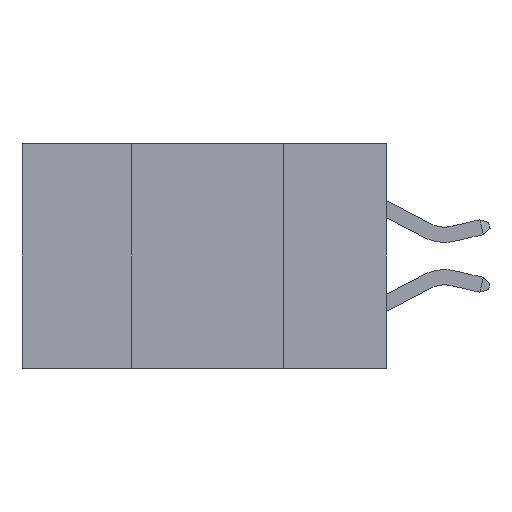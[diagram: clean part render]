
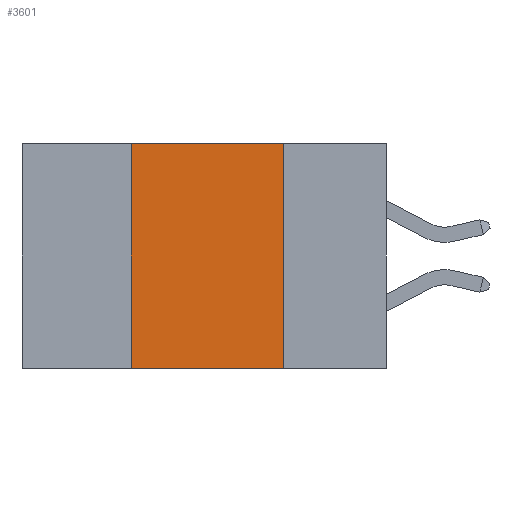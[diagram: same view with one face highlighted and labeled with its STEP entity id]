
A CAD part, left-side view. The second image highlights one B-rep face of the part: STEP entity #3601.
In plain terms, the highlighted planar face has unit normal (-1, 0, 0).
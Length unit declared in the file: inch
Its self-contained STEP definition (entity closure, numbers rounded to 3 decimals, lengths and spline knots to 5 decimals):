
#58 = DIRECTION ( 'NONE',  ( 0., 0., 1. ) ) ;
#184 = VERTEX_POINT ( 'NONE', #14784 ) ;
#425 = VERTEX_POINT ( 'NONE', #8489 ) ;
#799 = DIRECTION ( 'NONE',  ( 0., -1., 0. ) ) ;
#1236 = DIRECTION ( 'NONE',  ( 1., 0., 0. ) ) ;
#2021 = CARTESIAN_POINT ( 'NONE',  ( 0., 0.17, -0.37 ) ) ;
#2344 = VECTOR ( 'NONE', #799, 39.37008 ) ;
#3211 = ORIENTED_EDGE ( 'NONE', *, *, #11657, .T. ) ;
#3601 = ADVANCED_FACE ( 'NONE', ( #13585 ), #10010, .F. ) ;
#3607 = EDGE_CURVE ( 'NONE', #425, #15676, #8582, .T. ) ;
#3729 = DIRECTION ( 'NONE',  ( 0., 0., -1. ) ) ;
#4873 = EDGE_CURVE ( 'NONE', #184, #13789, #9852, .T. ) ;
#6885 = EDGE_CURVE ( 'NONE', #15676, #184, #9037, .T. ) ;
#7059 = ORIENTED_EDGE ( 'NONE', *, *, #4873, .F. ) ;
#7981 = CARTESIAN_POINT ( 'NONE',  ( 0., 0.6, 0. ) ) ;
#8489 = CARTESIAN_POINT ( 'NONE',  ( 0., 0.42, -0.37 ) ) ;
#8582 = LINE ( 'NONE', #8653, #11221 ) ;
#8603 = DIRECTION ( 'NONE',  ( 0., -1., 0. ) ) ;
#8653 = CARTESIAN_POINT ( 'NONE',  ( 0., 0.42, -0.37 ) ) ;
#8711 = ORIENTED_EDGE ( 'NONE', *, *, #3607, .F. ) ;
#9037 = LINE ( 'NONE', #7981, #2344 ) ;
#9701 = AXIS2_PLACEMENT_3D ( 'NONE', #9858, #1236, #3729 ) ;
#9702 = DIRECTION ( 'NONE',  ( 0., 0., -1. ) ) ;
#9852 = LINE ( 'NONE', #12387, #14281 ) ;
#9858 = CARTESIAN_POINT ( 'NONE',  ( 0., 0.6, 0. ) ) ;
#10010 = PLANE ( 'NONE',  #9701 ) ;
#11221 = VECTOR ( 'NONE', #58, 39.37008 ) ;
#11343 = ORIENTED_EDGE ( 'NONE', *, *, #6885, .F. ) ;
#11657 = EDGE_CURVE ( 'NONE', #425, #13789, #14661, .T. ) ;
#12387 = CARTESIAN_POINT ( 'NONE',  ( 0., 0.17, -0.37 ) ) ;
#13135 = EDGE_LOOP ( 'NONE', ( #7059, #11343, #8711, #3211 ) ) ;
#13585 = FACE_OUTER_BOUND ( 'NONE', #13135, .T. ) ;
#13789 = VERTEX_POINT ( 'NONE', #2021 ) ;
#14029 = CARTESIAN_POINT ( 'NONE',  ( 0., 0.42, 0. ) ) ;
#14106 = VECTOR ( 'NONE', #8603, 39.37008 ) ;
#14281 = VECTOR ( 'NONE', #9702, 39.37008 ) ;
#14661 = LINE ( 'NONE', #14737, #14106 ) ;
#14737 = CARTESIAN_POINT ( 'NONE',  ( 0., 0.6, -0.37 ) ) ;
#14784 = CARTESIAN_POINT ( 'NONE',  ( 0., 0.17, 0. ) ) ;
#15676 = VERTEX_POINT ( 'NONE', #14029 ) ;
